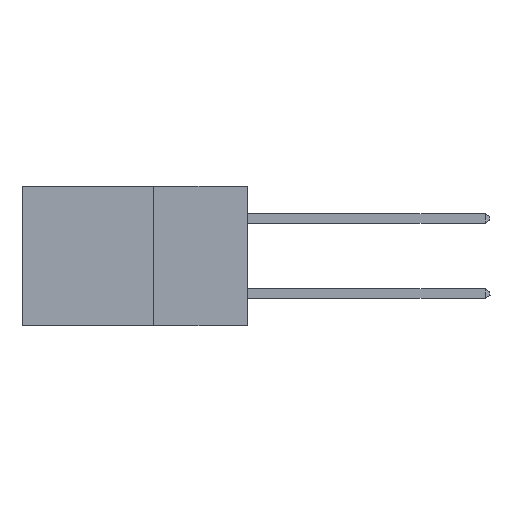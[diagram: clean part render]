
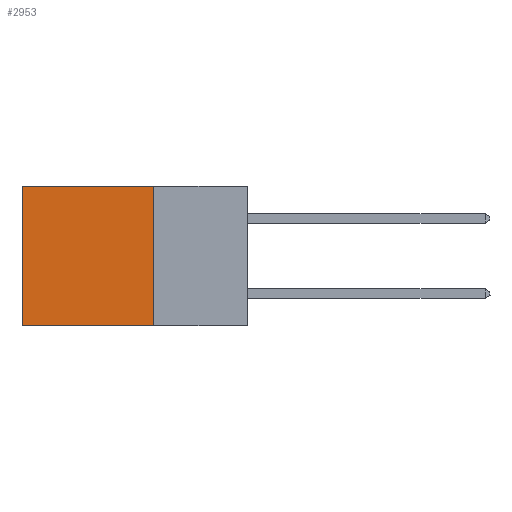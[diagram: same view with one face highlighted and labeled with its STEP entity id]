
A CAD part, left-side view. The second image highlights one B-rep face of the part: STEP entity #2953.
In plain terms, the highlighted planar face has unit normal (-1, 0, 0).
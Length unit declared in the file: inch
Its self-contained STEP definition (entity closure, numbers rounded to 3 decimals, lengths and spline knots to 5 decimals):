
#475 = VECTOR ( 'NONE', #10536, 39.37008 ) ;
#1253 = CARTESIAN_POINT ( 'NONE',  ( 0.298, 0.6, 0. ) ) ;
#1444 = EDGE_LOOP ( 'NONE', ( #11503, #1803, #8226, #3786 ) ) ;
#1611 = VERTEX_POINT ( 'NONE', #3845 ) ;
#1625 = FACE_OUTER_BOUND ( 'NONE', #1444, .T. ) ;
#1803 = ORIENTED_EDGE ( 'NONE', *, *, #5783, .F. ) ;
#2315 = LINE ( 'NONE', #4007, #4051 ) ;
#2387 = EDGE_CURVE ( 'NONE', #1611, #7352, #5632, .T. ) ;
#2953 = ADVANCED_FACE ( 'NONE', ( #1625 ), #4482, .F. ) ;
#3344 = DIRECTION ( 'NONE',  ( 0., 0., -1. ) ) ;
#3465 = CARTESIAN_POINT ( 'NONE',  ( 0.298, 0.25, -0.37 ) ) ;
#3786 = ORIENTED_EDGE ( 'NONE', *, *, #10762, .T. ) ;
#3845 = CARTESIAN_POINT ( 'NONE',  ( 0.298, 0.6, 0. ) ) ;
#4007 = CARTESIAN_POINT ( 'NONE',  ( 0.298, 0.25, 0. ) ) ;
#4051 = VECTOR ( 'NONE', #5502, 39.37008 ) ;
#4309 = AXIS2_PLACEMENT_3D ( 'NONE', #8454, #5533, #4452 ) ;
#4452 = DIRECTION ( 'NONE',  ( 0., 0., -1. ) ) ;
#4482 = PLANE ( 'NONE',  #4309 ) ;
#5302 = VECTOR ( 'NONE', #3344, 39.37008 ) ;
#5502 = DIRECTION ( 'NONE',  ( 0., 1., 0. ) ) ;
#5533 = DIRECTION ( 'NONE',  ( 1., 0., 0. ) ) ;
#5632 = LINE ( 'NONE', #1253, #5302 ) ;
#5675 = LINE ( 'NONE', #10595, #6446 ) ;
#5783 = EDGE_CURVE ( 'NONE', #7398, #7352, #13073, .T. ) ;
#6446 = VECTOR ( 'NONE', #7369, 39.37008 ) ;
#7352 = VERTEX_POINT ( 'NONE', #7388 ) ;
#7369 = DIRECTION ( 'NONE',  ( 0., 0., -1. ) ) ;
#7388 = CARTESIAN_POINT ( 'NONE',  ( 0.298, 0.6, -0.37 ) ) ;
#7398 = VERTEX_POINT ( 'NONE', #11592 ) ;
#8226 = ORIENTED_EDGE ( 'NONE', *, *, #10411, .F. ) ;
#8454 = CARTESIAN_POINT ( 'NONE',  ( 0.298, 0.25, 0. ) ) ;
#9372 = VERTEX_POINT ( 'NONE', #13142 ) ;
#10411 = EDGE_CURVE ( 'NONE', #9372, #7398, #5675, .T. ) ;
#10536 = DIRECTION ( 'NONE',  ( 0., 1., 0. ) ) ;
#10595 = CARTESIAN_POINT ( 'NONE',  ( 0.298, 0.25, 0. ) ) ;
#10762 = EDGE_CURVE ( 'NONE', #9372, #1611, #2315, .T. ) ;
#11503 = ORIENTED_EDGE ( 'NONE', *, *, #2387, .T. ) ;
#11592 = CARTESIAN_POINT ( 'NONE',  ( 0.298, 0.25, -0.37 ) ) ;
#13073 = LINE ( 'NONE', #3465, #475 ) ;
#13142 = CARTESIAN_POINT ( 'NONE',  ( 0.298, 0.25, 0. ) ) ;
